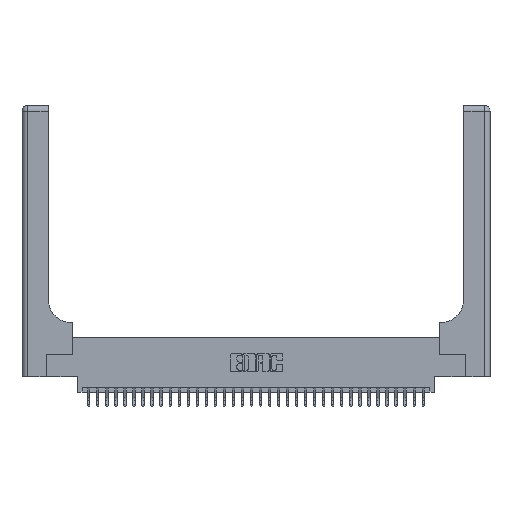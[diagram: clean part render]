
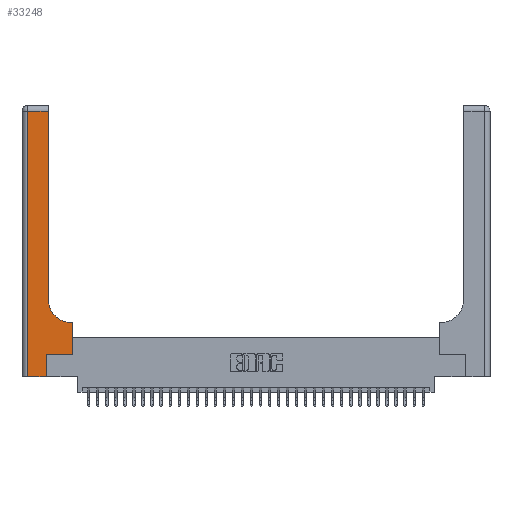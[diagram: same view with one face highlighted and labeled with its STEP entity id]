
A CAD part, top view. The second image highlights one B-rep face of the part: STEP entity #33248.
In plain terms, the highlighted planar face has unit normal (0, 0, 1).
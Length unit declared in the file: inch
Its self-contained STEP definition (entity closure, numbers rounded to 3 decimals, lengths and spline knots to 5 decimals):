
#9 = ORIENTED_EDGE ( 'NONE', *, *, #11028, .T. ) ;
#495 = CARTESIAN_POINT ( 'NONE',  ( 0.2915, 0.85, 0.37 ) ) ;
#889 = DIRECTION ( 'NONE',  ( 0., 1., 0. ) ) ;
#1412 = EDGE_CURVE ( 'NONE', #31219, #31769, #24989, .T. ) ;
#1556 = DIRECTION ( 'NONE',  ( 1., 0., 0. ) ) ;
#3296 = VECTOR ( 'NONE', #33002, 39.37008 ) ;
#3767 = DIRECTION ( 'NONE',  ( -1., 0., 0. ) ) ;
#4042 = LINE ( 'NONE', #25516, #7059 ) ;
#4060 = CARTESIAN_POINT ( 'NONE',  ( 0.269, 0., 0.37 ) ) ;
#4134 = ORIENTED_EDGE ( 'NONE', *, *, #30166, .T. ) ;
#4592 = CARTESIAN_POINT ( 'NONE',  ( 0., 3., 0.37 ) ) ;
#5346 = VECTOR ( 'NONE', #3767, 39.37008 ) ;
#5642 = LINE ( 'NONE', #24988, #23359 ) ;
#6307 = ORIENTED_EDGE ( 'NONE', *, *, #16886, .T. ) ;
#6844 = DIRECTION ( 'NONE',  ( 0., 0., -1. ) ) ;
#7059 = VECTOR ( 'NONE', #9124, 39.37008 ) ;
#7202 = DIRECTION ( 'NONE',  ( 0., 0., -1. ) ) ;
#7891 = CIRCLE ( 'NONE', #24126, 0.25 ) ;
#8057 = LINE ( 'NONE', #29186, #21916 ) ;
#9124 = DIRECTION ( 'NONE',  ( 0., 1., 0. ) ) ;
#9429 = CARTESIAN_POINT ( 'NONE',  ( 0., 0., 0.37 ) ) ;
#9576 = VERTEX_POINT ( 'NONE', #24481 ) ;
#9612 = VERTEX_POINT ( 'NONE', #21895 ) ;
#9657 = EDGE_CURVE ( 'NONE', #23111, #23059, #4042, .T. ) ;
#10527 = VERTEX_POINT ( 'NONE', #33193 ) ;
#10553 = ORIENTED_EDGE ( 'NONE', *, *, #21564, .T. ) ;
#10846 = CARTESIAN_POINT ( 'NONE',  ( 0., 2.94, 0.37 ) ) ;
#11028 = EDGE_CURVE ( 'NONE', #9576, #23111, #18294, .T. ) ;
#11934 = CARTESIAN_POINT ( 'NONE',  ( 0.5585, 0.25, 0.37 ) ) ;
#13005 = DIRECTION ( 'NONE',  ( -1., 0., 0. ) ) ;
#13654 = VERTEX_POINT ( 'NONE', #35486 ) ;
#15847 = VECTOR ( 'NONE', #23234, 39.37008 ) ;
#16886 = EDGE_CURVE ( 'NONE', #32147, #9612, #5642, .T. ) ;
#16976 = LINE ( 'NONE', #10846, #24845 ) ;
#17743 = ORIENTED_EDGE ( 'NONE', *, *, #1412, .T. ) ;
#18294 = LINE ( 'NONE', #32458, #24846 ) ;
#18334 = CARTESIAN_POINT ( 'NONE',  ( 0.5415, 0.85, 0.37 ) ) ;
#18748 = EDGE_CURVE ( 'NONE', #13654, #31219, #8057, .T. ) ;
#19290 = LINE ( 'NONE', #20563, #15847 ) ;
#20563 = CARTESIAN_POINT ( 'NONE',  ( 0.269, 0., 0.37 ) ) ;
#21564 = EDGE_CURVE ( 'NONE', #9612, #13654, #16976, .T. ) ;
#21895 = CARTESIAN_POINT ( 'NONE',  ( 0.2915, 2.94, 0.37 ) ) ;
#21916 = VECTOR ( 'NONE', #23197, 39.37008 ) ;
#22088 = EDGE_CURVE ( 'NONE', #10527, #32147, #7891, .T. ) ;
#23059 = VERTEX_POINT ( 'NONE', #31047 ) ;
#23111 = VERTEX_POINT ( 'NONE', #11934 ) ;
#23197 = DIRECTION ( 'NONE',  ( 0., -1., 0. ) ) ;
#23234 = DIRECTION ( 'NONE',  ( 0., 1., 0. ) ) ;
#23359 = VECTOR ( 'NONE', #889, 39.37008 ) ;
#24126 = AXIS2_PLACEMENT_3D ( 'NONE', #18334, #6844, #29029 ) ;
#24398 = ORIENTED_EDGE ( 'NONE', *, *, #22088, .T. ) ;
#24440 = CARTESIAN_POINT ( 'NONE',  ( 0.06, 0., 0.37 ) ) ;
#24481 = CARTESIAN_POINT ( 'NONE',  ( 0.269, 0.25, 0.37 ) ) ;
#24820 = LINE ( 'NONE', #28589, #5346 ) ;
#24845 = VECTOR ( 'NONE', #32892, 39.37008 ) ;
#24846 = VECTOR ( 'NONE', #1556, 39.37008 ) ;
#24988 = CARTESIAN_POINT ( 'NONE',  ( 0.2915, 3., 0.37 ) ) ;
#24989 = LINE ( 'NONE', #9429, #3296 ) ;
#25022 = ORIENTED_EDGE ( 'NONE', *, *, #26008, .T. ) ;
#25039 = AXIS2_PLACEMENT_3D ( 'NONE', #4592, #7202, #13005 ) ;
#25408 = ORIENTED_EDGE ( 'NONE', *, *, #9657, .T. ) ;
#25516 = CARTESIAN_POINT ( 'NONE',  ( 0.5585, 0.25, 0.37 ) ) ;
#26008 = EDGE_CURVE ( 'NONE', #23059, #10527, #24820, .T. ) ;
#27073 = ORIENTED_EDGE ( 'NONE', *, *, #18748, .T. ) ;
#28589 = CARTESIAN_POINT ( 'NONE',  ( 0.2915, 0.6, 0.37 ) ) ;
#29029 = DIRECTION ( 'NONE',  ( 1., 0., 0. ) ) ;
#29186 = CARTESIAN_POINT ( 'NONE',  ( 0.06, 3., 0.37 ) ) ;
#29287 = PLANE ( 'NONE',  #25039 ) ;
#30166 = EDGE_CURVE ( 'NONE', #31769, #9576, #19290, .T. ) ;
#31047 = CARTESIAN_POINT ( 'NONE',  ( 0.5585, 0.6, 0.37 ) ) ;
#31219 = VERTEX_POINT ( 'NONE', #24440 ) ;
#31769 = VERTEX_POINT ( 'NONE', #4060 ) ;
#32147 = VERTEX_POINT ( 'NONE', #495 ) ;
#32458 = CARTESIAN_POINT ( 'NONE',  ( 0.269, 0.25, 0.37 ) ) ;
#32659 = FACE_OUTER_BOUND ( 'NONE', #33242, .T. ) ;
#32892 = DIRECTION ( 'NONE',  ( -1., 0., 0. ) ) ;
#33002 = DIRECTION ( 'NONE',  ( 1., 0., 0. ) ) ;
#33193 = CARTESIAN_POINT ( 'NONE',  ( 0.5415, 0.6, 0.37 ) ) ;
#33242 = EDGE_LOOP ( 'NONE', ( #6307, #10553, #27073, #17743, #4134, #9, #25408, #25022, #24398 ) ) ;
#33248 = ADVANCED_FACE ( 'NONE', ( #32659 ), #29287, .F. ) ;
#35486 = CARTESIAN_POINT ( 'NONE',  ( 0.06, 2.94, 0.37 ) ) ;
